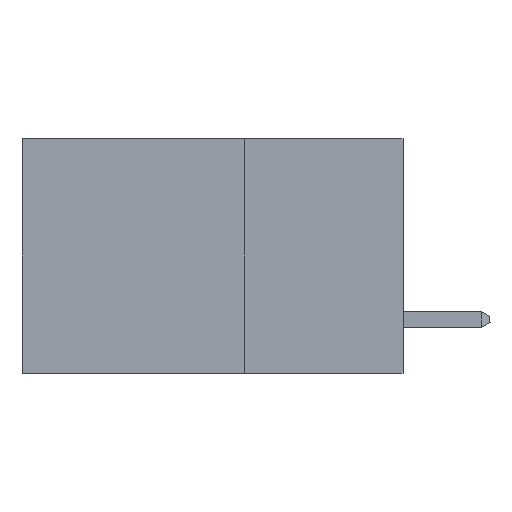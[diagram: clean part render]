
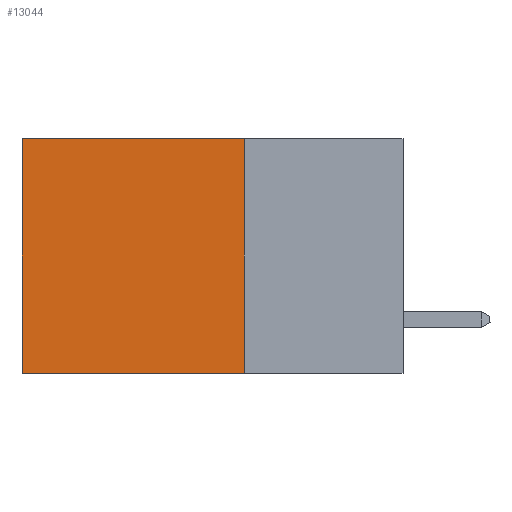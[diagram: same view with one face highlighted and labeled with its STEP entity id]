
A CAD part, left-side view. The second image highlights one B-rep face of the part: STEP entity #13044.
In plain terms, the highlighted planar face has unit normal (-1, 0, 0).
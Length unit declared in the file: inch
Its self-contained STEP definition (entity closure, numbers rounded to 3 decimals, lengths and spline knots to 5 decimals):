
#1856 = ORIENTED_EDGE ( 'NONE', *, *, #15240, .T. ) ;
#2901 = CARTESIAN_POINT ( 'NONE',  ( 0.2875, 0.6, 0. ) ) ;
#3692 = CARTESIAN_POINT ( 'NONE',  ( 0.2875, 0.25, 0. ) ) ;
#3836 = VERTEX_POINT ( 'NONE', #8873 ) ;
#4750 = VECTOR ( 'NONE', #14436, 39.37008 ) ;
#5170 = VECTOR ( 'NONE', #23986, 39.37008 ) ;
#5407 = LINE ( 'NONE', #26149, #24411 ) ;
#5482 = CARTESIAN_POINT ( 'NONE',  ( 0.2875, 0.25, -0.37 ) ) ;
#5758 = CARTESIAN_POINT ( 'NONE',  ( 0.2875, 0.6, -0.37 ) ) ;
#7415 = VECTOR ( 'NONE', #24556, 39.37008 ) ;
#7453 = ORIENTED_EDGE ( 'NONE', *, *, #32266, .T. ) ;
#7458 = VERTEX_POINT ( 'NONE', #5482 ) ;
#8233 = ORIENTED_EDGE ( 'NONE', *, *, #29061, .F. ) ;
#8554 = EDGE_CURVE ( 'NONE', #7458, #32411, #22492, .T. ) ;
#8873 = CARTESIAN_POINT ( 'NONE',  ( 0.2875, 0.25, 0. ) ) ;
#9874 = LINE ( 'NONE', #15017, #7415 ) ;
#10926 = AXIS2_PLACEMENT_3D ( 'NONE', #3692, #29928, #22458 ) ;
#12546 = DIRECTION ( 'NONE',  ( 0., 0., -1. ) ) ;
#13044 = ADVANCED_FACE ( 'NONE', ( #33535 ), #22106, .F. ) ;
#14436 = DIRECTION ( 'NONE',  ( 0., 1., 0. ) ) ;
#15017 = CARTESIAN_POINT ( 'NONE',  ( 0.2875, 0.25, 0. ) ) ;
#15240 = EDGE_CURVE ( 'NONE', #3836, #30438, #9874, .T. ) ;
#15898 = LINE ( 'NONE', #2901, #5170 ) ;
#18613 = ORIENTED_EDGE ( 'NONE', *, *, #8554, .F. ) ;
#22106 = PLANE ( 'NONE',  #10926 ) ;
#22458 = DIRECTION ( 'NONE',  ( 0., 0., -1. ) ) ;
#22492 = LINE ( 'NONE', #27570, #4750 ) ;
#23986 = DIRECTION ( 'NONE',  ( 0., 0., -1. ) ) ;
#24411 = VECTOR ( 'NONE', #12546, 39.37008 ) ;
#24556 = DIRECTION ( 'NONE',  ( 0., 1., 0. ) ) ;
#26149 = CARTESIAN_POINT ( 'NONE',  ( 0.2875, 0.25, 0. ) ) ;
#27570 = CARTESIAN_POINT ( 'NONE',  ( 0.2875, 0.25, -0.37 ) ) ;
#29061 = EDGE_CURVE ( 'NONE', #3836, #7458, #5407, .T. ) ;
#29928 = DIRECTION ( 'NONE',  ( 1., 0., 0. ) ) ;
#30438 = VERTEX_POINT ( 'NONE', #32218 ) ;
#31983 = EDGE_LOOP ( 'NONE', ( #7453, #18613, #8233, #1856 ) ) ;
#32218 = CARTESIAN_POINT ( 'NONE',  ( 0.2875, 0.6, 0. ) ) ;
#32266 = EDGE_CURVE ( 'NONE', #30438, #32411, #15898, .T. ) ;
#32411 = VERTEX_POINT ( 'NONE', #5758 ) ;
#33535 = FACE_OUTER_BOUND ( 'NONE', #31983, .T. ) ;
